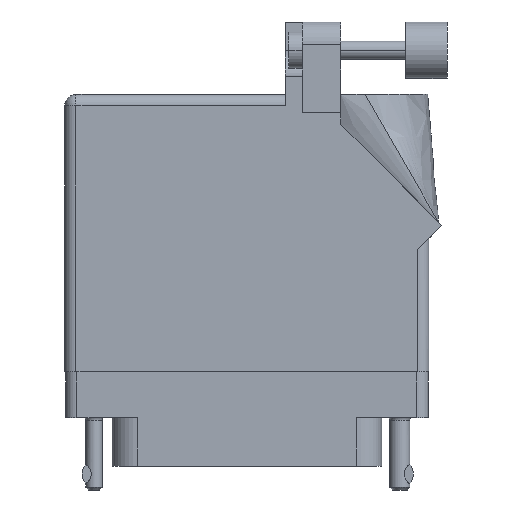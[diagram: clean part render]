
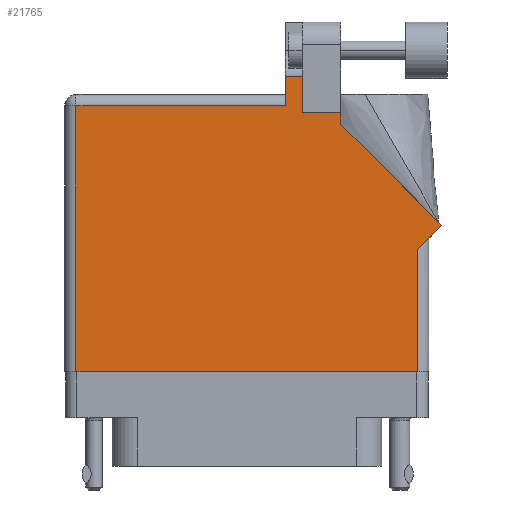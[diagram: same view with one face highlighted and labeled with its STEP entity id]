
A CAD part, front view. The second image highlights one B-rep face of the part: STEP entity #21765.
In plain terms, the highlighted face is planar.
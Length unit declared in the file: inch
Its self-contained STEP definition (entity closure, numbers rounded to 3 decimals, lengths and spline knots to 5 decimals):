
#149 = EDGE_CURVE ( 'NONE', #34444, #42399, #44605, .T. ) ;
#2263 = CARTESIAN_POINT ( 'NONE',  ( 0.306, 1.33, 0.455 ) ) ;
#2281 = CARTESIAN_POINT ( 'NONE',  ( 0.519, 1.26442, 0.455 ) ) ;
#2604 = CARTESIAN_POINT ( 'NONE',  ( 0.212, 1.368, 0.455 ) ) ;
#2776 = VECTOR ( 'NONE', #43115, 39.37008 ) ;
#3481 = DIRECTION ( 'NONE',  ( 0., 1., 0. ) ) ;
#3484 = DIRECTION ( 'NONE',  ( 0., 0., -1. ) ) ;
#4682 = DIRECTION ( 'NONE',  ( 1., 0., 0. ) ) ;
#5975 = VERTEX_POINT ( 'NONE', #29080 ) ;
#6447 = ORIENTED_EDGE ( 'NONE', *, *, #34741, .T. ) ;
#6504 = ORIENTED_EDGE ( 'NONE', *, *, #23188, .T. ) ;
#7182 = LINE ( 'NONE', #2281, #35912 ) ;
#8364 = VECTOR ( 'NONE', #28433, 39.37008 ) ;
#9605 = CARTESIAN_POINT ( 'NONE',  ( 1.07571, 0.70771, 0.455 ) ) ;
#11650 = CARTESIAN_POINT ( 'NONE',  ( -1.005, -0.1, 0.455 ) ) ;
#11725 = LINE ( 'NONE', #31307, #32162 ) ;
#12015 = EDGE_CURVE ( 'NONE', #18832, #38139, #30041, .T. ) ;
#12061 = ORIENTED_EDGE ( 'NONE', *, *, #32370, .T. ) ;
#12358 = VECTOR ( 'NONE', #35445, 39.37008 ) ;
#12706 = EDGE_CURVE ( 'NONE', #42399, #29410, #11725, .T. ) ;
#12743 = VERTEX_POINT ( 'NONE', #2604 ) ;
#13155 = CARTESIAN_POINT ( 'NONE',  ( 1.005, 0.637, 0.455 ) ) ;
#13472 = ORIENTED_EDGE ( 'NONE', *, *, #33287, .T. ) ;
#13989 = LINE ( 'NONE', #24613, #12358 ) ;
#14554 = CARTESIAN_POINT ( 'NONE',  ( -1.005, 1.43, 0.455 ) ) ;
#15806 = VERTEX_POINT ( 'NONE', #28919 ) ;
#16889 = LINE ( 'NONE', #11650, #22438 ) ;
#17814 = CARTESIAN_POINT ( 'NONE',  ( 0.943, 0.637, 0.455 ) ) ;
#18402 = VECTOR ( 'NONE', #34166, 39.37008 ) ;
#18832 = VERTEX_POINT ( 'NONE', #26485 ) ;
#19171 = CARTESIAN_POINT ( 'NONE',  ( -0.943, -0.1, 0.455 ) ) ;
#20429 = ORIENTED_EDGE ( 'NONE', *, *, #30015, .T. ) ;
#21613 = LINE ( 'NONE', #39648, #8364 ) ;
#21765 = ADVANCED_FACE ( 'NONE', ( #36563 ), #25066, .F. ) ;
#22438 = VECTOR ( 'NONE', #4682, 39.37008 ) ;
#22759 = LINE ( 'NONE', #17814, #35999 ) ;
#23188 = EDGE_CURVE ( 'NONE', #12743, #5975, #25369, .T. ) ;
#23711 = CARTESIAN_POINT ( 'NONE',  ( -0.943, -0.1, 0.455 ) ) ;
#24200 = ORIENTED_EDGE ( 'NONE', *, *, #35285, .T. ) ;
#24613 = CARTESIAN_POINT ( 'NONE',  ( 0.519, 1.33, 0.455 ) ) ;
#24843 = CARTESIAN_POINT ( 'NONE',  ( 1.07571, 0.70771, 0.455 ) ) ;
#24994 = CARTESIAN_POINT ( 'NONE',  ( 0.943, -0.1, 0.455 ) ) ;
#25066 = PLANE ( 'NONE',  #39010 ) ;
#25369 = LINE ( 'NONE', #32461, #2776 ) ;
#25451 = VERTEX_POINT ( 'NONE', #33074 ) ;
#26485 = CARTESIAN_POINT ( 'NONE',  ( 0.943, 0.575, 0.455 ) ) ;
#26682 = ORIENTED_EDGE ( 'NONE', *, *, #12706, .T. ) ;
#28433 = DIRECTION ( 'NONE',  ( 0., -1., 0. ) ) ;
#28592 = EDGE_CURVE ( 'NONE', #25451, #34444, #13989, .T. ) ;
#28691 = CARTESIAN_POINT ( 'NONE',  ( 0.306, 1.5315, 0.455 ) ) ;
#28919 = CARTESIAN_POINT ( 'NONE',  ( 0.519, 1.26442, 0.455 ) ) ;
#29080 = CARTESIAN_POINT ( 'NONE',  ( -0.943, 1.368, 0.455 ) ) ;
#29410 = VERTEX_POINT ( 'NONE', #36600 ) ;
#30015 = EDGE_CURVE ( 'NONE', #45312, #18832, #22759, .T. ) ;
#30041 = LINE ( 'NONE', #13155, #18402 ) ;
#30720 = DIRECTION ( 'NONE',  ( -1., 0., 0. ) ) ;
#31307 = CARTESIAN_POINT ( 'NONE',  ( 0.63677, 1.5315, 0.455 ) ) ;
#31971 = DIRECTION ( 'NONE',  ( -0.707, 0.707, 0. ) ) ;
#32162 = VECTOR ( 'NONE', #30720, 39.37008 ) ;
#32370 = EDGE_CURVE ( 'NONE', #5975, #36195, #43000, .T. ) ;
#32461 = CARTESIAN_POINT ( 'NONE',  ( -1.005, 1.368, 0.455 ) ) ;
#32997 = VECTOR ( 'NONE', #41983, 39.37008 ) ;
#33074 = CARTESIAN_POINT ( 'NONE',  ( 0.519, 1.33, 0.455 ) ) ;
#33287 = EDGE_CURVE ( 'NONE', #38139, #15806, #44036, .T. ) ;
#34166 = DIRECTION ( 'NONE',  ( 0.707, 0.707, 0. ) ) ;
#34444 = VERTEX_POINT ( 'NONE', #2263 ) ;
#34634 = VECTOR ( 'NONE', #31971, 39.37008 ) ;
#34741 = EDGE_CURVE ( 'NONE', #36195, #45312, #16889, .T. ) ;
#35285 = EDGE_CURVE ( 'NONE', #29410, #12743, #21613, .T. ) ;
#35445 = DIRECTION ( 'NONE',  ( -1., 0., 0. ) ) ;
#35912 = VECTOR ( 'NONE', #36855, 39.37008 ) ;
#35999 = VECTOR ( 'NONE', #3481, 39.37008 ) ;
#36195 = VERTEX_POINT ( 'NONE', #19171 ) ;
#36563 = FACE_OUTER_BOUND ( 'NONE', #44192, .T. ) ;
#36600 = CARTESIAN_POINT ( 'NONE',  ( 0.212, 1.5315, 0.455 ) ) ;
#36855 = DIRECTION ( 'NONE',  ( 0., 1., 0. ) ) ;
#38034 = ORIENTED_EDGE ( 'NONE', *, *, #149, .T. ) ;
#38139 = VERTEX_POINT ( 'NONE', #9605 ) ;
#38659 = DIRECTION ( 'NONE',  ( -1., 0., 0. ) ) ;
#38856 = CARTESIAN_POINT ( 'NONE',  ( 0.306, 1.33, 0.455 ) ) ;
#39010 = AXIS2_PLACEMENT_3D ( 'NONE', #14554, #3484, #38659 ) ;
#39263 = ORIENTED_EDGE ( 'NONE', *, *, #43693, .T. ) ;
#39648 = CARTESIAN_POINT ( 'NONE',  ( 0.212, 1.43, 0.455 ) ) ;
#39896 = ORIENTED_EDGE ( 'NONE', *, *, #12015, .T. ) ;
#40170 = VECTOR ( 'NONE', #45027, 39.37008 ) ;
#41983 = DIRECTION ( 'NONE',  ( 0., 1., 0. ) ) ;
#42399 = VERTEX_POINT ( 'NONE', #28691 ) ;
#43000 = LINE ( 'NONE', #23711, #40170 ) ;
#43115 = DIRECTION ( 'NONE',  ( -1., 0., 0. ) ) ;
#43693 = EDGE_CURVE ( 'NONE', #15806, #25451, #7182, .T. ) ;
#44036 = LINE ( 'NONE', #24843, #34634 ) ;
#44192 = EDGE_LOOP ( 'NONE', ( #38034, #26682, #24200, #6504, #12061, #6447, #20429, #39896, #13472, #39263, #44764 ) ) ;
#44605 = LINE ( 'NONE', #38856, #32997 ) ;
#44764 = ORIENTED_EDGE ( 'NONE', *, *, #28592, .T. ) ;
#45027 = DIRECTION ( 'NONE',  ( 0., -1., 0. ) ) ;
#45312 = VERTEX_POINT ( 'NONE', #24994 ) ;
